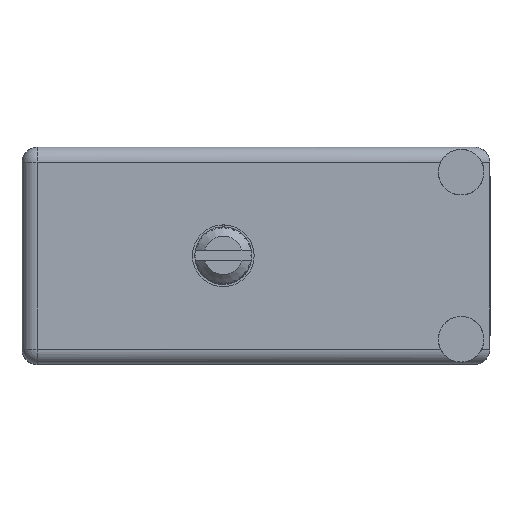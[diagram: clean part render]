
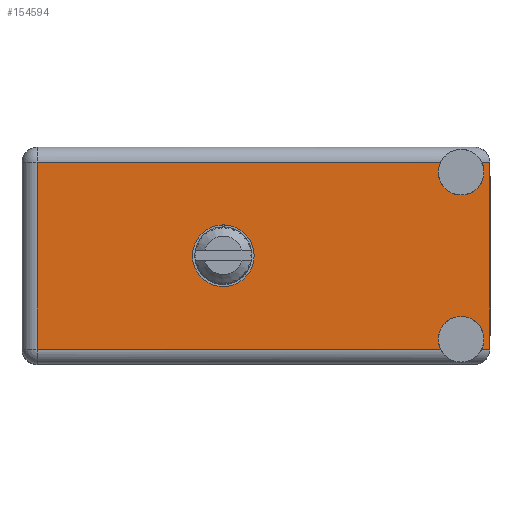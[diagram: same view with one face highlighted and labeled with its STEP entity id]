
A CAD part, top view. The second image highlights one B-rep face of the part: STEP entity #154594.
In plain terms, the highlighted face is planar.
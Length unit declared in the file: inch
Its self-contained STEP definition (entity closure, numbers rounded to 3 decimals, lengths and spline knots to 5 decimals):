
#2222 = LINE ( 'NONE', #161889, #155793 ) ;
#4569 = EDGE_CURVE ( 'NONE', #56132, #127575, #149927, .T. ) ;
#5298 = CIRCLE ( 'NONE', #49132, 0.1015 ) ;
#6353 = DIRECTION ( 'NONE',  ( 0., 0., 1. ) ) ;
#7929 = CARTESIAN_POINT ( 'NONE',  ( 1.51259, 0.906, -0.05 ) ) ;
#8619 = AXIS2_PLACEMENT_3D ( 'NONE', #38100, #192417, #85701 ) ;
#11710 = DIRECTION ( 'NONE',  ( 0., 0., 1. ) ) ;
#12274 = ORIENTED_EDGE ( 'NONE', *, *, #104145, .T. ) ;
#13614 = VERTEX_POINT ( 'NONE', #179317 ) ;
#16443 = CARTESIAN_POINT ( 'NONE',  ( 1.539, 0.906, -0.665 ) ) ;
#16602 = EDGE_LOOP ( 'NONE', ( #98780, #19172, #17895, #47954, #50165, #90541, #37887, #156312, #167163, #12274 ) ) ;
#17895 = ORIENTED_EDGE ( 'NONE', *, *, #46766, .F. ) ;
#19172 = ORIENTED_EDGE ( 'NONE', *, *, #19518, .F. ) ;
#19518 = EDGE_CURVE ( 'NONE', #13614, #187599, #175365, .T. ) ;
#19668 = CIRCLE ( 'NONE', #63253, 0.075 ) ;
#20792 = CARTESIAN_POINT ( 'NONE',  ( 0.6625, 0.906, -0.3575 ) ) ;
#21325 = CARTESIAN_POINT ( 'NONE',  ( 1.37741, 0.906, -0.05 ) ) ;
#21792 = DIRECTION ( 'NONE',  ( 0., 1., 0. ) ) ;
#22794 = VERTEX_POINT ( 'NONE', #7929 ) ;
#25632 = DIRECTION ( 'NONE',  ( 1., 0., 0. ) ) ;
#27763 = PLANE ( 'NONE',  #144244 ) ;
#29317 = CARTESIAN_POINT ( 'NONE',  ( 0.05, 0.906, -0.665 ) ) ;
#30589 = LINE ( 'NONE', #129333, #92939 ) ;
#32087 = EDGE_CURVE ( 'NONE', #74336, #118997, #78286, .T. ) ;
#37887 = ORIENTED_EDGE ( 'NONE', *, *, #62533, .F. ) ;
#38100 = CARTESIAN_POINT ( 'NONE',  ( 1.445, 0.906, -0.0825 ) ) ;
#41051 = CIRCLE ( 'NONE', #144774, 0.075 ) ;
#43809 = DIRECTION ( 'NONE',  ( 0., 1., 0. ) ) ;
#44700 = VERTEX_POINT ( 'NONE', #118945 ) ;
#46766 = EDGE_CURVE ( 'NONE', #22794, #13614, #182665, .T. ) ;
#47954 = ORIENTED_EDGE ( 'NONE', *, *, #113046, .T. ) ;
#49132 = AXIS2_PLACEMENT_3D ( 'NONE', #20792, #50228, #52230 ) ;
#50165 = ORIENTED_EDGE ( 'NONE', *, *, #4569, .F. ) ;
#50228 = DIRECTION ( 'NONE',  ( 0., 1., 0. ) ) ;
#50906 = AXIS2_PLACEMENT_3D ( 'NONE', #98225, #21792, #6353 ) ;
#52230 = DIRECTION ( 'NONE',  ( 0., 0., 1. ) ) ;
#53802 = CARTESIAN_POINT ( 'NONE',  ( 1.445, 0.906, -0.6325 ) ) ;
#56132 = VERTEX_POINT ( 'NONE', #16443 ) ;
#56741 = EDGE_CURVE ( 'NONE', #86187, #128423, #140197, .T. ) ;
#57412 = VERTEX_POINT ( 'NONE', #164120 ) ;
#58102 = CARTESIAN_POINT ( 'NONE',  ( 0.6625, 0.906, -0.3575 ) ) ;
#58765 = EDGE_CURVE ( 'NONE', #86187, #44700, #19668, .T. ) ;
#60564 = CARTESIAN_POINT ( 'NONE',  ( 1.51259, 0.906, -0.665 ) ) ;
#62533 = EDGE_CURVE ( 'NONE', #44700, #88263, #41051, .T. ) ;
#63253 = AXIS2_PLACEMENT_3D ( 'NONE', #53802, #99503, #176656 ) ;
#74336 = VERTEX_POINT ( 'NONE', #139480 ) ;
#78228 = EDGE_LOOP ( 'NONE', ( #100438, #81741 ) ) ;
#78286 = CIRCLE ( 'NONE', #89876, 0.1015 ) ;
#79165 = CARTESIAN_POINT ( 'NONE',  ( 0.6625, 0.906, -0.459 ) ) ;
#81741 = ORIENTED_EDGE ( 'NONE', *, *, #88809, .F. ) ;
#85701 = DIRECTION ( 'NONE',  ( 0., 0., 1. ) ) ;
#86187 = VERTEX_POINT ( 'NONE', #147032 ) ;
#88263 = VERTEX_POINT ( 'NONE', #60564 ) ;
#88809 = EDGE_CURVE ( 'NONE', #118997, #74336, #5298, .T. ) ;
#89876 = AXIS2_PLACEMENT_3D ( 'NONE', #58102, #182911, #165508 ) ;
#90541 = ORIENTED_EDGE ( 'NONE', *, *, #178111, .T. ) ;
#92939 = VECTOR ( 'NONE', #149336, 39.37008 ) ;
#93604 = DIRECTION ( 'NONE',  ( 0., 0., 1. ) ) ;
#96654 = CARTESIAN_POINT ( 'NONE',  ( 0., 0.906, -0.665 ) ) ;
#96659 = CARTESIAN_POINT ( 'NONE',  ( 1.539, 0.906, -0.05 ) ) ;
#98225 = CARTESIAN_POINT ( 'NONE',  ( 1.445, 0.906, -0.0825 ) ) ;
#98780 = ORIENTED_EDGE ( 'NONE', *, *, #109714, .T. ) ;
#99503 = DIRECTION ( 'NONE',  ( 0., 1., 0. ) ) ;
#100438 = ORIENTED_EDGE ( 'NONE', *, *, #32087, .F. ) ;
#104145 = EDGE_CURVE ( 'NONE', #128423, #57412, #108008, .T. ) ;
#104890 = CARTESIAN_POINT ( 'NONE',  ( 0., 0.906, -0.715 ) ) ;
#106596 = VECTOR ( 'NONE', #154282, 39.37008 ) ;
#108008 = LINE ( 'NONE', #158540, #170355 ) ;
#109714 = EDGE_CURVE ( 'NONE', #57412, #187599, #2222, .T. ) ;
#112351 = CARTESIAN_POINT ( 'NONE',  ( 1.539, 0.906, -0.05 ) ) ;
#113046 = EDGE_CURVE ( 'NONE', #22794, #127575, #122007, .T. ) ;
#118945 = CARTESIAN_POINT ( 'NONE',  ( 1.445, 0.906, -0.5575 ) ) ;
#118997 = VERTEX_POINT ( 'NONE', #79165 ) ;
#122007 = LINE ( 'NONE', #112351, #126828 ) ;
#123978 = FACE_OUTER_BOUND ( 'NONE', #16602, .T. ) ;
#126828 = VECTOR ( 'NONE', #143903, 39.37008 ) ;
#127575 = VERTEX_POINT ( 'NONE', #96659 ) ;
#128423 = VERTEX_POINT ( 'NONE', #29317 ) ;
#129333 = CARTESIAN_POINT ( 'NONE',  ( 0., 0.906, -0.665 ) ) ;
#139480 = CARTESIAN_POINT ( 'NONE',  ( 0.6625, 0.906, -0.256 ) ) ;
#140197 = LINE ( 'NONE', #96654, #176222 ) ;
#143903 = DIRECTION ( 'NONE',  ( 1., 0., 0. ) ) ;
#144244 = AXIS2_PLACEMENT_3D ( 'NONE', #104890, #43809, #11710 ) ;
#144774 = AXIS2_PLACEMENT_3D ( 'NONE', #154029, #169433, #93604 ) ;
#147032 = CARTESIAN_POINT ( 'NONE',  ( 1.37741, 0.906, -0.665 ) ) ;
#149336 = DIRECTION ( 'NONE',  ( -1., 0., 0. ) ) ;
#149927 = LINE ( 'NONE', #187099, #106596 ) ;
#152816 = FACE_BOUND ( 'NONE', #78228, .T. ) ;
#154029 = CARTESIAN_POINT ( 'NONE',  ( 1.445, 0.906, -0.6325 ) ) ;
#154282 = DIRECTION ( 'NONE',  ( 0., 0., 1. ) ) ;
#154594 = ADVANCED_FACE ( 'NONE', ( #152816, #123978 ), #27763, .T. ) ;
#155793 = VECTOR ( 'NONE', #25632, 39.37008 ) ;
#156312 = ORIENTED_EDGE ( 'NONE', *, *, #58765, .F. ) ;
#158540 = CARTESIAN_POINT ( 'NONE',  ( 0.05, 0.906, -0.715 ) ) ;
#161889 = CARTESIAN_POINT ( 'NONE',  ( 1.539, 0.906, -0.05 ) ) ;
#164120 = CARTESIAN_POINT ( 'NONE',  ( 0.05, 0.906, -0.05 ) ) ;
#165508 = DIRECTION ( 'NONE',  ( 0., 0., 1. ) ) ;
#167163 = ORIENTED_EDGE ( 'NONE', *, *, #56741, .T. ) ;
#169433 = DIRECTION ( 'NONE',  ( 0., 1., 0. ) ) ;
#170355 = VECTOR ( 'NONE', #175300, 39.37008 ) ;
#175300 = DIRECTION ( 'NONE',  ( 0., 0., 1. ) ) ;
#175365 = CIRCLE ( 'NONE', #50906, 0.075 ) ;
#176222 = VECTOR ( 'NONE', #185908, 39.37008 ) ;
#176656 = DIRECTION ( 'NONE',  ( 0., 0., 1. ) ) ;
#178111 = EDGE_CURVE ( 'NONE', #56132, #88263, #30589, .T. ) ;
#179317 = CARTESIAN_POINT ( 'NONE',  ( 1.445, 0.906, -0.1575 ) ) ;
#182665 = CIRCLE ( 'NONE', #8619, 0.075 ) ;
#182911 = DIRECTION ( 'NONE',  ( 0., 1., 0. ) ) ;
#185908 = DIRECTION ( 'NONE',  ( -1., 0., 0. ) ) ;
#187099 = CARTESIAN_POINT ( 'NONE',  ( 1.539, 0.906, 0. ) ) ;
#187599 = VERTEX_POINT ( 'NONE', #21325 ) ;
#192417 = DIRECTION ( 'NONE',  ( 0., 1., 0. ) ) ;
